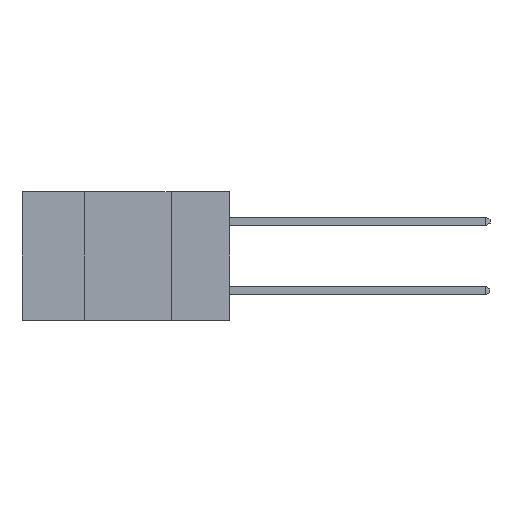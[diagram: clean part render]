
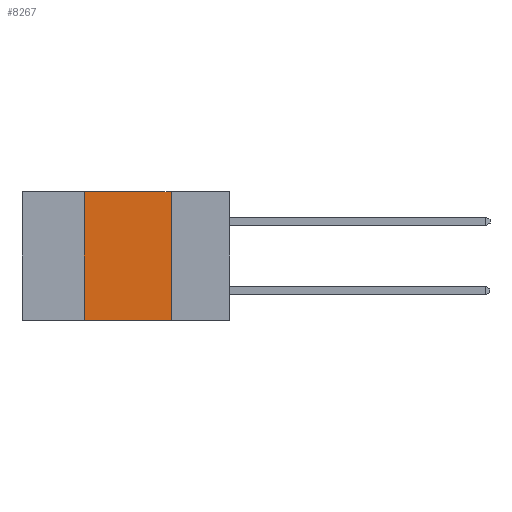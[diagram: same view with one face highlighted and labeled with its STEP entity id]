
A CAD part, left-side view. The second image highlights one B-rep face of the part: STEP entity #8267.
In plain terms, the highlighted planar face has unit normal (-1, 0, 0).
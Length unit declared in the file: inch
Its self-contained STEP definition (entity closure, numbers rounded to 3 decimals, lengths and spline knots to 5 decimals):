
#887 = LINE ( 'NONE', #1227, #7453 ) ;
#915 = EDGE_CURVE ( 'NONE', #8456, #10751, #7872, .T. ) ;
#1059 = VECTOR ( 'NONE', #4951, 39.37008 ) ;
#1171 = ORIENTED_EDGE ( 'NONE', *, *, #915, .F. ) ;
#1194 = CARTESIAN_POINT ( 'NONE',  ( 0., 0.17, 0. ) ) ;
#1227 = CARTESIAN_POINT ( 'NONE',  ( 0., 0.6, -0.37 ) ) ;
#1446 = ORIENTED_EDGE ( 'NONE', *, *, #7941, .F. ) ;
#1768 = VERTEX_POINT ( 'NONE', #2147 ) ;
#1782 = DIRECTION ( 'NONE',  ( 0., 0., -1. ) ) ;
#1823 = VECTOR ( 'NONE', #3754, 39.37008 ) ;
#2147 = CARTESIAN_POINT ( 'NONE',  ( 0., 0.42, -0.37 ) ) ;
#2263 = DIRECTION ( 'NONE',  ( 0., -1., 0. ) ) ;
#2641 = VECTOR ( 'NONE', #2263, 39.37008 ) ;
#3528 = EDGE_CURVE ( 'NONE', #1768, #7049, #8860, .T. ) ;
#3754 = DIRECTION ( 'NONE',  ( 0., 0., 1. ) ) ;
#3801 = CARTESIAN_POINT ( 'NONE',  ( 0., 0.42, 0. ) ) ;
#3836 = EDGE_LOOP ( 'NONE', ( #1171, #1446, #4178, #3976 ) ) ;
#3976 = ORIENTED_EDGE ( 'NONE', *, *, #10726, .T. ) ;
#4178 = ORIENTED_EDGE ( 'NONE', *, *, #3528, .F. ) ;
#4951 = DIRECTION ( 'NONE',  ( 0., 0., -1. ) ) ;
#5365 = CARTESIAN_POINT ( 'NONE',  ( 0., 0.6, 0. ) ) ;
#5395 = AXIS2_PLACEMENT_3D ( 'NONE', #5365, #7154, #1782 ) ;
#5705 = DIRECTION ( 'NONE',  ( 0., -1., 0. ) ) ;
#5850 = CARTESIAN_POINT ( 'NONE',  ( 0., 0.6, 0. ) ) ;
#6266 = PLANE ( 'NONE',  #5395 ) ;
#6709 = FACE_OUTER_BOUND ( 'NONE', #3836, .T. ) ;
#7049 = VERTEX_POINT ( 'NONE', #8313 ) ;
#7154 = DIRECTION ( 'NONE',  ( 1., 0., 0. ) ) ;
#7453 = VECTOR ( 'NONE', #5705, 39.37008 ) ;
#7659 = CARTESIAN_POINT ( 'NONE',  ( 0., 0.17, 0. ) ) ;
#7872 = LINE ( 'NONE', #7659, #1059 ) ;
#7941 = EDGE_CURVE ( 'NONE', #7049, #8456, #9361, .T. ) ;
#8267 = ADVANCED_FACE ( 'NONE', ( #6709 ), #6266, .F. ) ;
#8313 = CARTESIAN_POINT ( 'NONE',  ( 0., 0.42, 0. ) ) ;
#8456 = VERTEX_POINT ( 'NONE', #1194 ) ;
#8860 = LINE ( 'NONE', #3801, #1823 ) ;
#9361 = LINE ( 'NONE', #5850, #2641 ) ;
#10031 = CARTESIAN_POINT ( 'NONE',  ( 0., 0.17, -0.37 ) ) ;
#10726 = EDGE_CURVE ( 'NONE', #1768, #10751, #887, .T. ) ;
#10751 = VERTEX_POINT ( 'NONE', #10031 ) ;
